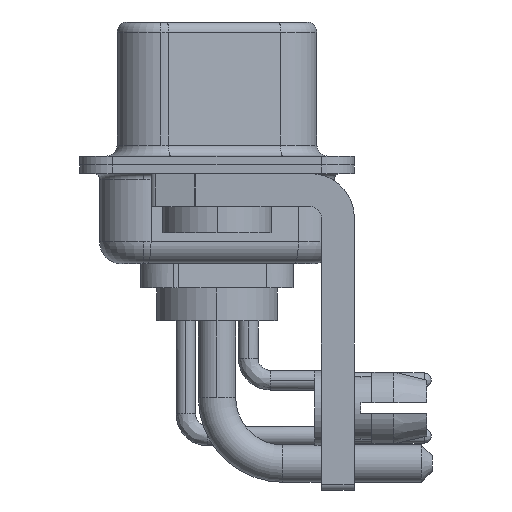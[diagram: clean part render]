
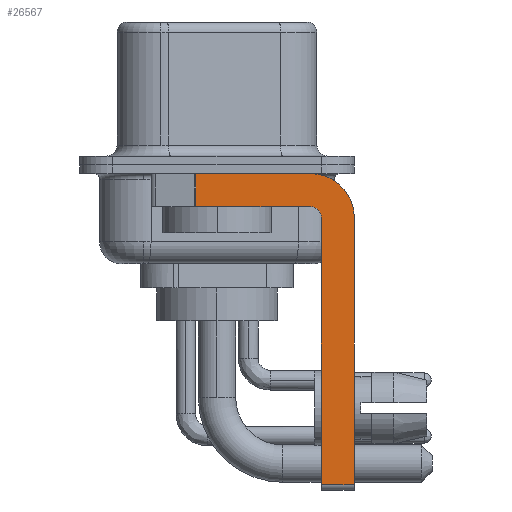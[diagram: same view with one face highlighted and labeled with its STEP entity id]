
A CAD part, left-side view. The second image highlights one B-rep face of the part: STEP entity #26567.
In plain terms, the highlighted planar face has unit normal (-1, 0, 0).
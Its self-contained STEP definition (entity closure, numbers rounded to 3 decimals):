
#239 = VECTOR ( 'NONE', #9536, 1000. ) ;
#752 = CARTESIAN_POINT ( 'NONE',  ( -2.9, -4.25, -1.9 ) ) ;
#2358 = EDGE_CURVE ( 'NONE', #23173, #17991, #26492, .T. ) ;
#2493 = CIRCLE ( 'NONE', #18437, 0.5 ) ;
#2528 = DIRECTION ( 'NONE',  ( 0., -1., 0. ) ) ;
#2635 = CARTESIAN_POINT ( 'NONE',  ( -2.9, 0.978, -1.9 ) ) ;
#2944 = DIRECTION ( 'NONE',  ( 0., 0., -1. ) ) ;
#3351 = VERTEX_POINT ( 'NONE', #8069 ) ;
#4216 = CARTESIAN_POINT ( 'NONE',  ( -2.9, -6.25, -2.4 ) ) ;
#5140 = CARTESIAN_POINT ( 'NONE',  ( -2.9, -4.25, -2.4 ) ) ;
#5557 = DIRECTION ( 'NONE',  ( 0., -1., 0. ) ) ;
#5601 = EDGE_CURVE ( 'NONE', #24078, #3351, #19898, .T. ) ;
#6373 = EDGE_CURVE ( 'NONE', #9119, #25889, #15861, .T. ) ;
#7080 = DIRECTION ( 'NONE',  ( -1., 0., 0. ) ) ;
#7191 = CARTESIAN_POINT ( 'NONE',  ( -2.9, -6.25, -2.4 ) ) ;
#7668 = CARTESIAN_POINT ( 'NONE',  ( -2.9, -4.25, -0.4 ) ) ;
#8069 = CARTESIAN_POINT ( 'NONE',  ( -2.9, 0.978, -1.9 ) ) ;
#8199 = VECTOR ( 'NONE', #26610, 1000. ) ;
#8236 = AXIS2_PLACEMENT_3D ( 'NONE', #14987, #23723, #19842 ) ;
#8329 = ORIENTED_EDGE ( 'NONE', *, *, #5601, .T. ) ;
#8523 = ORIENTED_EDGE ( 'NONE', *, *, #27839, .F. ) ;
#8616 = EDGE_CURVE ( 'NONE', #25889, #19331, #2493, .T. ) ;
#8708 = CIRCLE ( 'NONE', #8236, 2. ) ;
#9119 = VERTEX_POINT ( 'NONE', #12265 ) ;
#9201 = DIRECTION ( 'NONE',  ( 0., 0., 1. ) ) ;
#9536 = DIRECTION ( 'NONE',  ( 0., 1., 0. ) ) ;
#9633 = EDGE_CURVE ( 'NONE', #9119, #17991, #20842, .T. ) ;
#10100 = ORIENTED_EDGE ( 'NONE', *, *, #8616, .F. ) ;
#10493 = EDGE_LOOP ( 'NONE', ( #15474, #8329, #8523, #10100, #24675, #14223, #11924, #20642 ) ) ;
#11924 = ORIENTED_EDGE ( 'NONE', *, *, #2358, .F. ) ;
#12231 = VECTOR ( 'NONE', #13701, 1000. ) ;
#12265 = CARTESIAN_POINT ( 'NONE',  ( -2.9, -4.75, -14.55 ) ) ;
#12513 = CARTESIAN_POINT ( 'NONE',  ( -2.9, -4.25, -14.55 ) ) ;
#13338 = CARTESIAN_POINT ( 'NONE',  ( -2.9, 3., -0.4 ) ) ;
#13701 = DIRECTION ( 'NONE',  ( 0., 0., 1. ) ) ;
#13840 = LINE ( 'NONE', #752, #239 ) ;
#13930 = CARTESIAN_POINT ( 'NONE',  ( -2.9, -4.25, -2.4 ) ) ;
#13974 = PLANE ( 'NONE',  #21658 ) ;
#14223 = ORIENTED_EDGE ( 'NONE', *, *, #9633, .T. ) ;
#14855 = EDGE_CURVE ( 'NONE', #24078, #21296, #24096, .T. ) ;
#14987 = CARTESIAN_POINT ( 'NONE',  ( -2.9, -4.25, -2.4 ) ) ;
#15474 = ORIENTED_EDGE ( 'NONE', *, *, #14855, .F. ) ;
#15565 = CARTESIAN_POINT ( 'NONE',  ( -2.9, -4.25, -1.9 ) ) ;
#15861 = LINE ( 'NONE', #22730, #12231 ) ;
#15954 = VECTOR ( 'NONE', #2528, 1000. ) ;
#16679 = VECTOR ( 'NONE', #5557, 1000. ) ;
#17194 = CARTESIAN_POINT ( 'NONE',  ( -2.9, -4.75, -2.4 ) ) ;
#17991 = VERTEX_POINT ( 'NONE', #24816 ) ;
#18437 = AXIS2_PLACEMENT_3D ( 'NONE', #13930, #7080, #9201 ) ;
#19325 = VECTOR ( 'NONE', #2944, 1000. ) ;
#19331 = VERTEX_POINT ( 'NONE', #15565 ) ;
#19842 = DIRECTION ( 'NONE',  ( 0., 0., -1. ) ) ;
#19898 = LINE ( 'NONE', #2635, #8199 ) ;
#20642 = ORIENTED_EDGE ( 'NONE', *, *, #23670, .F. ) ;
#20842 = LINE ( 'NONE', #12513, #16679 ) ;
#21296 = VERTEX_POINT ( 'NONE', #7668 ) ;
#21658 = AXIS2_PLACEMENT_3D ( 'NONE', #5140, #22292, #22432 ) ;
#22292 = DIRECTION ( 'NONE',  ( 1., 0., 0. ) ) ;
#22432 = DIRECTION ( 'NONE',  ( 0., 0., -1. ) ) ;
#22579 = FACE_OUTER_BOUND ( 'NONE', #10493, .T. ) ;
#22730 = CARTESIAN_POINT ( 'NONE',  ( -2.9, -4.75, -14.8 ) ) ;
#23173 = VERTEX_POINT ( 'NONE', #4216 ) ;
#23670 = EDGE_CURVE ( 'NONE', #21296, #23173, #8708, .T. ) ;
#23723 = DIRECTION ( 'NONE',  ( 1., 0., 0. ) ) ;
#24078 = VERTEX_POINT ( 'NONE', #24114 ) ;
#24096 = LINE ( 'NONE', #13338, #15954 ) ;
#24114 = CARTESIAN_POINT ( 'NONE',  ( -2.9, 0.978, -0.4 ) ) ;
#24675 = ORIENTED_EDGE ( 'NONE', *, *, #6373, .F. ) ;
#24816 = CARTESIAN_POINT ( 'NONE',  ( -2.9, -6.25, -14.55 ) ) ;
#25889 = VERTEX_POINT ( 'NONE', #17194 ) ;
#26492 = LINE ( 'NONE', #7191, #19325 ) ;
#26567 = ADVANCED_FACE ( 'NONE', ( #22579 ), #13974, .F. ) ;
#26610 = DIRECTION ( 'NONE',  ( 0., 0., -1. ) ) ;
#27839 = EDGE_CURVE ( 'NONE', #19331, #3351, #13840, .T. ) ;
